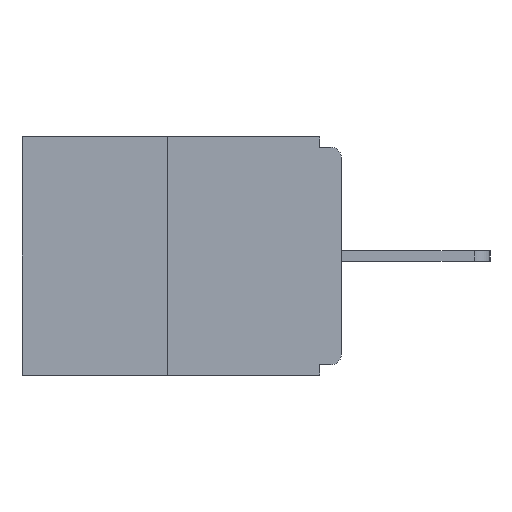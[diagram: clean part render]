
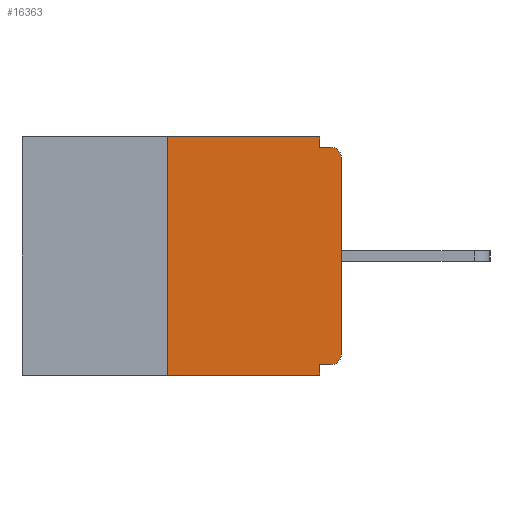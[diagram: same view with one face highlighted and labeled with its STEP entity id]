
A CAD part, left-side view. The second image highlights one B-rep face of the part: STEP entity #16363.
In plain terms, the highlighted planar face has unit normal (-1, 0, 0).
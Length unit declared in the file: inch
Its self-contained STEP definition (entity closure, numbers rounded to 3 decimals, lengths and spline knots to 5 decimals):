
#326 = PLANE ( 'NONE',  #1489 ) ;
#454 = VERTEX_POINT ( 'NONE', #22639 ) ;
#1230 = CARTESIAN_POINT ( 'NONE',  ( 0., 0.015, -0.015 ) ) ;
#1444 = CARTESIAN_POINT ( 'NONE',  ( 0., 0.031, 0. ) ) ;
#1489 = AXIS2_PLACEMENT_3D ( 'NONE', #12502, #8308, #16594 ) ;
#2168 = VERTEX_POINT ( 'NONE', #23254 ) ;
#2690 = LINE ( 'NONE', #22746, #17459 ) ;
#2744 = CARTESIAN_POINT ( 'NONE',  ( 0., 0., 0. ) ) ;
#3367 = VERTEX_POINT ( 'NONE', #17508 ) ;
#3585 = VECTOR ( 'NONE', #25100, 39.37008 ) ;
#3750 = LINE ( 'NONE', #5686, #19204 ) ;
#3820 = VERTEX_POINT ( 'NONE', #19708 ) ;
#4497 = CIRCLE ( 'NONE', #5763, 0.015 ) ;
#4684 = DIRECTION ( 'NONE',  ( -1., 0., 0. ) ) ;
#4883 = LINE ( 'NONE', #22850, #3585 ) ;
#5248 = EDGE_CURVE ( 'NONE', #24259, #24300, #20711, .T. ) ;
#5315 = VERTEX_POINT ( 'NONE', #1444 ) ;
#5686 = CARTESIAN_POINT ( 'NONE',  ( 0., 0.031, -0.343 ) ) ;
#5744 = CARTESIAN_POINT ( 'NONE',  ( 0., 0.46, 0. ) ) ;
#5763 = AXIS2_PLACEMENT_3D ( 'NONE', #8633, #4684, #19027 ) ;
#6016 = VECTOR ( 'NONE', #12699, 39.37008 ) ;
#6155 = AXIS2_PLACEMENT_3D ( 'NONE', #11913, #10070, #18367 ) ;
#6343 = DIRECTION ( 'NONE',  ( 0., 0., 1. ) ) ;
#6805 = CARTESIAN_POINT ( 'NONE',  ( 0., 0., -0.313 ) ) ;
#6936 = CARTESIAN_POINT ( 'NONE',  ( 0., 0.031, 0. ) ) ;
#7107 = CARTESIAN_POINT ( 'NONE',  ( 0., 0., -0.015 ) ) ;
#7641 = LINE ( 'NONE', #21186, #14321 ) ;
#7706 = DIRECTION ( 'NONE',  ( 0., -1., 0. ) ) ;
#8109 = EDGE_CURVE ( 'NONE', #3820, #3367, #4883, .T. ) ;
#8308 = DIRECTION ( 'NONE',  ( 1., 0., 0. ) ) ;
#8570 = FACE_OUTER_BOUND ( 'NONE', #17447, .T. ) ;
#8633 = CARTESIAN_POINT ( 'NONE',  ( 0., 0.015, -0.03 ) ) ;
#9223 = LINE ( 'NONE', #7107, #25306 ) ;
#9232 = ORIENTED_EDGE ( 'NONE', *, *, #8109, .T. ) ;
#9807 = ORIENTED_EDGE ( 'NONE', *, *, #14349, .F. ) ;
#10070 = DIRECTION ( 'NONE',  ( -1., 0., 0. ) ) ;
#10257 = EDGE_CURVE ( 'NONE', #3820, #454, #2690, .T. ) ;
#10740 = DIRECTION ( 'NONE',  ( 0., 0., 1. ) ) ;
#11403 = ORIENTED_EDGE ( 'NONE', *, *, #22110, .T. ) ;
#11477 = DIRECTION ( 'NONE',  ( 0., 1., 0. ) ) ;
#11527 = ORIENTED_EDGE ( 'NONE', *, *, #17418, .F. ) ;
#11913 = CARTESIAN_POINT ( 'NONE',  ( 0., 0.015, -0.313 ) ) ;
#12502 = CARTESIAN_POINT ( 'NONE',  ( 0., 0.46, 0. ) ) ;
#12699 = DIRECTION ( 'NONE',  ( 0., 0., -1. ) ) ;
#12755 = ORIENTED_EDGE ( 'NONE', *, *, #21564, .F. ) ;
#12776 = VERTEX_POINT ( 'NONE', #14219 ) ;
#12976 = CARTESIAN_POINT ( 'NONE',  ( 0., 0.015, -0.328 ) ) ;
#14058 = DIRECTION ( 'NONE',  ( 0., 0., -1. ) ) ;
#14219 = CARTESIAN_POINT ( 'NONE',  ( 0., 0.031, -0.015 ) ) ;
#14321 = VECTOR ( 'NONE', #11477, 39.37008 ) ;
#14349 = EDGE_CURVE ( 'NONE', #24275, #2168, #7641, .T. ) ;
#15726 = EDGE_CURVE ( 'NONE', #12776, #15804, #9223, .T. ) ;
#15804 = VERTEX_POINT ( 'NONE', #1230 ) ;
#16363 = ADVANCED_FACE ( 'NONE', ( #8570 ), #326, .F. ) ;
#16594 = DIRECTION ( 'NONE',  ( 0., 0., -1. ) ) ;
#17075 = LINE ( 'NONE', #6936, #6016 ) ;
#17101 = DIRECTION ( 'NONE',  ( 0., -1., 0. ) ) ;
#17335 = CARTESIAN_POINT ( 'NONE',  ( 0., 0., -0.03 ) ) ;
#17418 = EDGE_CURVE ( 'NONE', #5315, #12776, #17075, .T. ) ;
#17447 = EDGE_LOOP ( 'NONE', ( #17812, #20854, #9232, #12755, #9807, #25043, #24697, #11403, #22126, #11527 ) ) ;
#17459 = VECTOR ( 'NONE', #6343, 39.37008 ) ;
#17508 = CARTESIAN_POINT ( 'NONE',  ( 0., 0.031, -0.343 ) ) ;
#17717 = LINE ( 'NONE', #5744, #18701 ) ;
#17812 = ORIENTED_EDGE ( 'NONE', *, *, #25784, .F. ) ;
#18367 = DIRECTION ( 'NONE',  ( 0., 0., -1. ) ) ;
#18701 = VECTOR ( 'NONE', #7706, 39.37008 ) ;
#19027 = DIRECTION ( 'NONE',  ( 0., 0., -1. ) ) ;
#19204 = VECTOR ( 'NONE', #14058, 39.37008 ) ;
#19409 = VECTOR ( 'NONE', #10740, 39.37008 ) ;
#19708 = CARTESIAN_POINT ( 'NONE',  ( 0., 0.25, -0.343 ) ) ;
#20711 = LINE ( 'NONE', #2744, #19409 ) ;
#20854 = ORIENTED_EDGE ( 'NONE', *, *, #10257, .F. ) ;
#21186 = CARTESIAN_POINT ( 'NONE',  ( 0., 0., -0.328 ) ) ;
#21564 = EDGE_CURVE ( 'NONE', #2168, #3367, #3750, .T. ) ;
#21945 = EDGE_CURVE ( 'NONE', #24275, #24259, #25464, .T. ) ;
#22110 = EDGE_CURVE ( 'NONE', #24300, #15804, #4497, .T. ) ;
#22126 = ORIENTED_EDGE ( 'NONE', *, *, #15726, .F. ) ;
#22639 = CARTESIAN_POINT ( 'NONE',  ( 0., 0.25, 0. ) ) ;
#22746 = CARTESIAN_POINT ( 'NONE',  ( 0., 0.25, 0. ) ) ;
#22850 = CARTESIAN_POINT ( 'NONE',  ( 0., 0.46, -0.343 ) ) ;
#23254 = CARTESIAN_POINT ( 'NONE',  ( 0., 0.031, -0.328 ) ) ;
#24259 = VERTEX_POINT ( 'NONE', #6805 ) ;
#24275 = VERTEX_POINT ( 'NONE', #12976 ) ;
#24300 = VERTEX_POINT ( 'NONE', #17335 ) ;
#24697 = ORIENTED_EDGE ( 'NONE', *, *, #5248, .T. ) ;
#25043 = ORIENTED_EDGE ( 'NONE', *, *, #21945, .T. ) ;
#25100 = DIRECTION ( 'NONE',  ( 0., -1., 0. ) ) ;
#25306 = VECTOR ( 'NONE', #17101, 39.37008 ) ;
#25464 = CIRCLE ( 'NONE', #6155, 0.015 ) ;
#25784 = EDGE_CURVE ( 'NONE', #454, #5315, #17717, .T. ) ;
